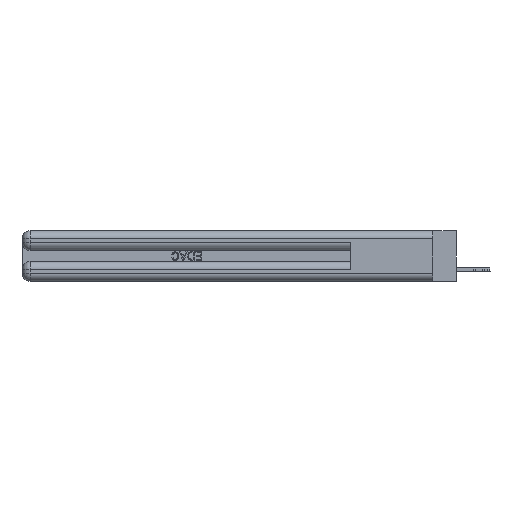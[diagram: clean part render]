
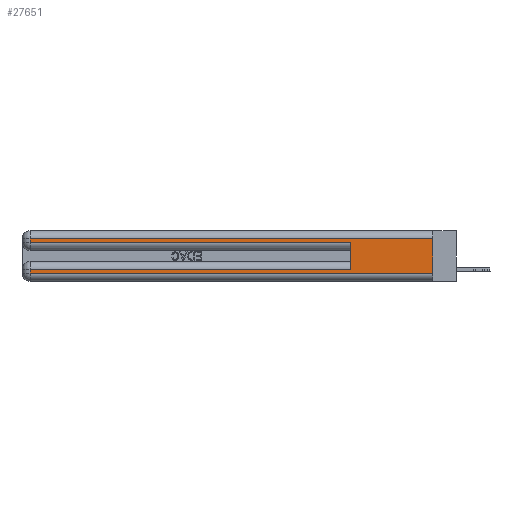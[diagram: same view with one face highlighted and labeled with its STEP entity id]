
A CAD part, left-side view. The second image highlights one B-rep face of the part: STEP entity #27651.
In plain terms, the highlighted planar face has unit normal (-1, 0, 0).
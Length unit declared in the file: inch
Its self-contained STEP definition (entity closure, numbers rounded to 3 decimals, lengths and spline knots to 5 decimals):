
#274 = EDGE_CURVE ( 'NONE', #29230, #3515, #27788, .T. ) ;
#756 = VERTEX_POINT ( 'NONE', #42618 ) ;
#1547 = VERTEX_POINT ( 'NONE', #3606 ) ;
#2004 = LINE ( 'NONE', #30667, #19958 ) ;
#2022 = PLANE ( 'NONE',  #15075 ) ;
#2305 = VECTOR ( 'NONE', #22339, 39.37008 ) ;
#2420 = EDGE_CURVE ( 'NONE', #29230, #28533, #37319, .T. ) ;
#2941 = CARTESIAN_POINT ( 'NONE',  ( 0., 0., 0.085 ) ) ;
#3207 = VERTEX_POINT ( 'NONE', #31278 ) ;
#3515 = VERTEX_POINT ( 'NONE', #29539 ) ;
#3606 = CARTESIAN_POINT ( 'NONE',  ( 0., 0., 0.31 ) ) ;
#4443 = DIRECTION ( 'NONE',  ( 0., 0., -1. ) ) ;
#4772 = VECTOR ( 'NONE', #7309, 39.37008 ) ;
#5023 = LINE ( 'NONE', #30919, #32686 ) ;
#5319 = EDGE_CURVE ( 'NONE', #19028, #3515, #2004, .T. ) ;
#5501 = DIRECTION ( 'NONE',  ( 0., 0., -1. ) ) ;
#5573 = ORIENTED_EDGE ( 'NONE', *, *, #8595, .T. ) ;
#6339 = LINE ( 'NONE', #14745, #40447 ) ;
#7017 = ORIENTED_EDGE ( 'NONE', *, *, #18928, .T. ) ;
#7309 = DIRECTION ( 'NONE',  ( 0., 1., 0. ) ) ;
#8595 = EDGE_CURVE ( 'NONE', #3207, #35374, #5023, .T. ) ;
#9734 = EDGE_CURVE ( 'NONE', #1547, #35374, #27030, .T. ) ;
#11979 = CARTESIAN_POINT ( 'NONE',  ( 0., 0., 0.37 ) ) ;
#14233 = ORIENTED_EDGE ( 'NONE', *, *, #274, .F. ) ;
#14745 = CARTESIAN_POINT ( 'NONE',  ( 0., 2.94, 0.37 ) ) ;
#14834 = CARTESIAN_POINT ( 'NONE',  ( 0., 2.94, 0.085 ) ) ;
#14925 = EDGE_CURVE ( 'NONE', #1547, #756, #44595, .T. ) ;
#15075 = AXIS2_PLACEMENT_3D ( 'NONE', #16288, #33105, #40505 ) ;
#15450 = EDGE_LOOP ( 'NONE', ( #41427, #34466, #7017, #19877, #14233, #44559, #20549, #5573 ) ) ;
#16217 = EDGE_CURVE ( 'NONE', #28533, #3207, #40644, .T. ) ;
#16288 = CARTESIAN_POINT ( 'NONE',  ( 0., 0., 0.37 ) ) ;
#16572 = CARTESIAN_POINT ( 'NONE',  ( 0., 2.94, 0.285 ) ) ;
#17782 = VECTOR ( 'NONE', #5501, 39.37008 ) ;
#18928 = EDGE_CURVE ( 'NONE', #756, #19028, #6339, .T. ) ;
#19028 = VERTEX_POINT ( 'NONE', #16572 ) ;
#19877 = ORIENTED_EDGE ( 'NONE', *, *, #5319, .T. ) ;
#19958 = VECTOR ( 'NONE', #44063, 39.37008 ) ;
#20549 = ORIENTED_EDGE ( 'NONE', *, *, #16217, .T. ) ;
#22339 = DIRECTION ( 'NONE',  ( 0., 1., 0. ) ) ;
#23288 = VECTOR ( 'NONE', #39422, 39.37008 ) ;
#24099 = DIRECTION ( 'NONE',  ( 0., -1., 0. ) ) ;
#24805 = CARTESIAN_POINT ( 'NONE',  ( 0., 0., 0.31 ) ) ;
#25074 = VECTOR ( 'NONE', #38226, 39.37008 ) ;
#27030 = LINE ( 'NONE', #11979, #17782 ) ;
#27651 = ADVANCED_FACE ( 'NONE', ( #44072 ), #2022, .F. ) ;
#27788 = LINE ( 'NONE', #34333, #25074 ) ;
#28533 = VERTEX_POINT ( 'NONE', #14834 ) ;
#29230 = VERTEX_POINT ( 'NONE', #31522 ) ;
#29539 = CARTESIAN_POINT ( 'NONE',  ( 0., 0.6, 0.285 ) ) ;
#30667 = CARTESIAN_POINT ( 'NONE',  ( 0., 0., 0.285 ) ) ;
#30672 = CARTESIAN_POINT ( 'NONE',  ( 0., 0., 0.06 ) ) ;
#30919 = CARTESIAN_POINT ( 'NONE',  ( 0., 0., 0.06 ) ) ;
#31278 = CARTESIAN_POINT ( 'NONE',  ( 0., 2.94, 0.06 ) ) ;
#31522 = CARTESIAN_POINT ( 'NONE',  ( 0., 0.6, 0.085 ) ) ;
#32492 = CARTESIAN_POINT ( 'NONE',  ( 0., 2.94, 0.37 ) ) ;
#32686 = VECTOR ( 'NONE', #24099, 39.37008 ) ;
#33105 = DIRECTION ( 'NONE',  ( 1., 0., 0. ) ) ;
#34333 = CARTESIAN_POINT ( 'NONE',  ( 0., 0.6, 0.145 ) ) ;
#34466 = ORIENTED_EDGE ( 'NONE', *, *, #14925, .T. ) ;
#35374 = VERTEX_POINT ( 'NONE', #30672 ) ;
#37319 = LINE ( 'NONE', #2941, #4772 ) ;
#38226 = DIRECTION ( 'NONE',  ( 0., 0., 1. ) ) ;
#39422 = DIRECTION ( 'NONE',  ( 0., 0., -1. ) ) ;
#40447 = VECTOR ( 'NONE', #4443, 39.37008 ) ;
#40505 = DIRECTION ( 'NONE',  ( 0., 0., -1. ) ) ;
#40644 = LINE ( 'NONE', #32492, #23288 ) ;
#41427 = ORIENTED_EDGE ( 'NONE', *, *, #9734, .F. ) ;
#42618 = CARTESIAN_POINT ( 'NONE',  ( 0., 2.94, 0.31 ) ) ;
#44063 = DIRECTION ( 'NONE',  ( 0., -1., 0. ) ) ;
#44072 = FACE_OUTER_BOUND ( 'NONE', #15450, .T. ) ;
#44559 = ORIENTED_EDGE ( 'NONE', *, *, #2420, .T. ) ;
#44595 = LINE ( 'NONE', #24805, #2305 ) ;
